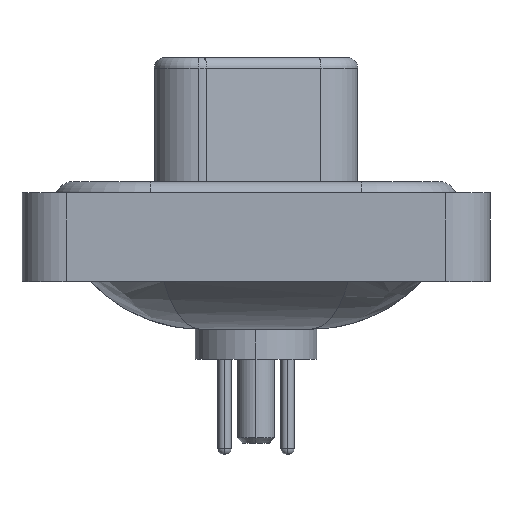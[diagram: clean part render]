
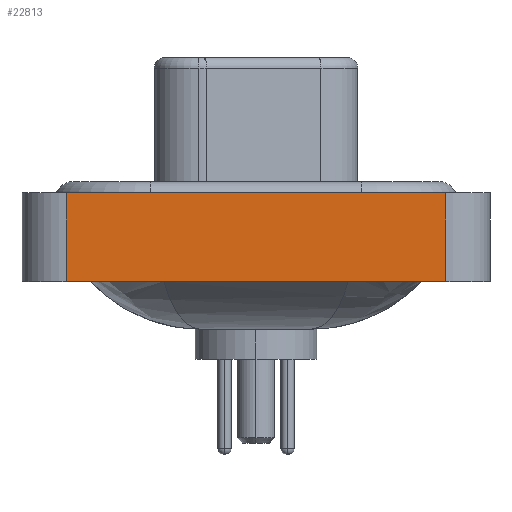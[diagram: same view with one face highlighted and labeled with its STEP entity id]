
A CAD part, left-side view. The second image highlights one B-rep face of the part: STEP entity #22813.
In plain terms, the highlighted planar face has unit normal (-1, 0, 0).
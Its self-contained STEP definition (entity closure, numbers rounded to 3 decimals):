
#475 = CARTESIAN_POINT ( 'NONE',  ( -7.35, -8.55, -3.6 ) ) ;
#1565 = DIRECTION ( 'NONE',  ( 0., -1., 0. ) ) ;
#1672 = VERTEX_POINT ( 'NONE', #21291 ) ;
#3686 = CARTESIAN_POINT ( 'NONE',  ( -7.35, -8.55, -3.6 ) ) ;
#4012 = VERTEX_POINT ( 'NONE', #8753 ) ;
#4546 = CARTESIAN_POINT ( 'NONE',  ( -7.35, 8.55, -3.6 ) ) ;
#5121 = EDGE_LOOP ( 'NONE', ( #5172, #21726, #21153, #18171 ) ) ;
#5168 = CARTESIAN_POINT ( 'NONE',  ( -7.35, -8.55, -3.6 ) ) ;
#5172 = ORIENTED_EDGE ( 'NONE', *, *, #21362, .T. ) ;
#5472 = LINE ( 'NONE', #12086, #12053 ) ;
#8753 = CARTESIAN_POINT ( 'NONE',  ( -7.35, -8.55, 0.4 ) ) ;
#8849 = EDGE_CURVE ( 'NONE', #10843, #4012, #5472, .T. ) ;
#9533 = DIRECTION ( 'NONE',  ( 0., 0., 1. ) ) ;
#9613 = AXIS2_PLACEMENT_3D ( 'NONE', #14762, #14987, #9533 ) ;
#9836 = CARTESIAN_POINT ( 'NONE',  ( -7.35, 8.55, 0.4 ) ) ;
#10218 = DIRECTION ( 'NONE',  ( 0., -1., 0. ) ) ;
#10843 = VERTEX_POINT ( 'NONE', #9836 ) ;
#11414 = DIRECTION ( 'NONE',  ( 0., 0., 1. ) ) ;
#11501 = PLANE ( 'NONE',  #9613 ) ;
#12053 = VECTOR ( 'NONE', #10218, 1000. ) ;
#12086 = CARTESIAN_POINT ( 'NONE',  ( -7.35, -8.55, 0.4 ) ) ;
#14757 = LINE ( 'NONE', #475, #15163 ) ;
#14762 = CARTESIAN_POINT ( 'NONE',  ( -7.35, -8.55, -3.6 ) ) ;
#14987 = DIRECTION ( 'NONE',  ( -1., 0., 0. ) ) ;
#15163 = VECTOR ( 'NONE', #20104, 1000. ) ;
#18171 = ORIENTED_EDGE ( 'NONE', *, *, #18792, .T. ) ;
#18792 = EDGE_CURVE ( 'NONE', #1672, #21852, #20975, .T. ) ;
#20104 = DIRECTION ( 'NONE',  ( 0., 0., 1. ) ) ;
#20259 = LINE ( 'NONE', #4546, #21093 ) ;
#20341 = FACE_OUTER_BOUND ( 'NONE', #5121, .T. ) ;
#20359 = VECTOR ( 'NONE', #1565, 1000. ) ;
#20975 = LINE ( 'NONE', #5168, #20359 ) ;
#21034 = EDGE_CURVE ( 'NONE', #1672, #10843, #20259, .T. ) ;
#21093 = VECTOR ( 'NONE', #11414, 1000. ) ;
#21153 = ORIENTED_EDGE ( 'NONE', *, *, #21034, .F. ) ;
#21291 = CARTESIAN_POINT ( 'NONE',  ( -7.35, 8.55, -3.6 ) ) ;
#21362 = EDGE_CURVE ( 'NONE', #21852, #4012, #14757, .T. ) ;
#21726 = ORIENTED_EDGE ( 'NONE', *, *, #8849, .F. ) ;
#21852 = VERTEX_POINT ( 'NONE', #3686 ) ;
#22813 = ADVANCED_FACE ( 'NONE', ( #20341 ), #11501, .T. ) ;
